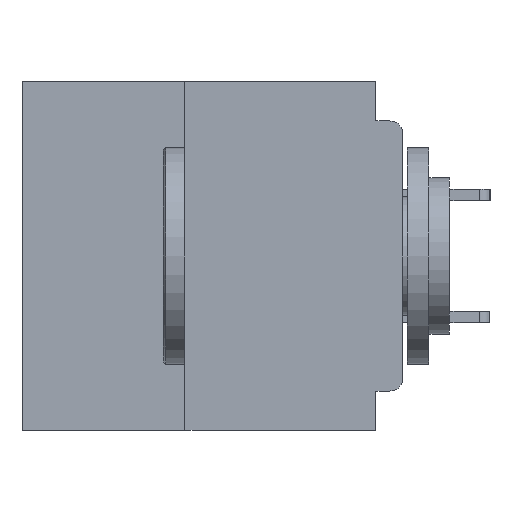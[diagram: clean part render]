
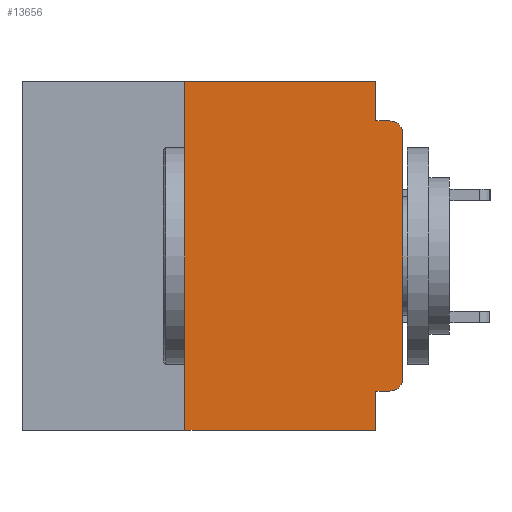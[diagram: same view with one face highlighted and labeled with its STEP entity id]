
A CAD part, left-side view. The second image highlights one B-rep face of the part: STEP entity #13656.
In plain terms, the highlighted planar face has unit normal (-1, 0, 0).
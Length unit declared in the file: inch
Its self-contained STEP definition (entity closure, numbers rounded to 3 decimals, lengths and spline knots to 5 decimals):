
#329 = EDGE_LOOP ( 'NONE', ( #6978, #16661, #8367, #24212, #28486, #1615, #40626, #20095, #39759, #20184 ) ) ;
#485 = LINE ( 'NONE', #35036, #35221 ) ;
#985 = VERTEX_POINT ( 'NONE', #24131 ) ;
#1359 = LINE ( 'NONE', #37734, #35083 ) ;
#1615 = ORIENTED_EDGE ( 'NONE', *, *, #29564, .F. ) ;
#3371 = CIRCLE ( 'NONE', #28947, 0.015 ) ;
#3474 = EDGE_CURVE ( 'NONE', #6209, #32710, #10884, .T. ) ;
#3659 = VERTEX_POINT ( 'NONE', #36518 ) ;
#3709 = DIRECTION ( 'NONE',  ( 0., -1., 0. ) ) ;
#4823 = CARTESIAN_POINT ( 'NONE',  ( 0., 0.437, 0. ) ) ;
#5097 = VECTOR ( 'NONE', #8752, 39.37008 ) ;
#5295 = PLANE ( 'NONE',  #34351 ) ;
#5691 = CARTESIAN_POINT ( 'NONE',  ( 0., 0.031, -0.045 ) ) ;
#5872 = CARTESIAN_POINT ( 'NONE',  ( 0., 0.015, -0.06 ) ) ;
#6209 = VERTEX_POINT ( 'NONE', #13935 ) ;
#6978 = ORIENTED_EDGE ( 'NONE', *, *, #35087, .T. ) ;
#7083 = CARTESIAN_POINT ( 'NONE',  ( 0., 0.015, -0.34 ) ) ;
#7646 = CARTESIAN_POINT ( 'NONE',  ( 0., 0.031, 0. ) ) ;
#8367 = ORIENTED_EDGE ( 'NONE', *, *, #11167, .F. ) ;
#8616 = CARTESIAN_POINT ( 'NONE',  ( 0., 0.031, -0.355 ) ) ;
#8752 = DIRECTION ( 'NONE',  ( 0., -1., 0. ) ) ;
#9049 = VECTOR ( 'NONE', #41411, 39.37008 ) ;
#9162 = DIRECTION ( 'NONE',  ( 0., 0., -1. ) ) ;
#10382 = DIRECTION ( 'NONE',  ( 0., 0., -1. ) ) ;
#10881 = EDGE_CURVE ( 'NONE', #29014, #27771, #3371, .T. ) ;
#10884 = LINE ( 'NONE', #4823, #35881 ) ;
#11167 = EDGE_CURVE ( 'NONE', #37117, #41996, #1359, .T. ) ;
#11799 = CARTESIAN_POINT ( 'NONE',  ( 0., 0.25, -0.4 ) ) ;
#11869 = DIRECTION ( 'NONE',  ( 0., 0., -1. ) ) ;
#13554 = FACE_OUTER_BOUND ( 'NONE', #329, .T. ) ;
#13656 = ADVANCED_FACE ( 'NONE', ( #13554 ), #5295, .F. ) ;
#13844 = LINE ( 'NONE', #40713, #38805 ) ;
#13924 = VECTOR ( 'NONE', #41183, 39.37008 ) ;
#13935 = CARTESIAN_POINT ( 'NONE',  ( 0., 0.25, 0. ) ) ;
#15252 = VECTOR ( 'NONE', #31895, 39.37008 ) ;
#16661 = ORIENTED_EDGE ( 'NONE', *, *, #30199, .T. ) ;
#17846 = EDGE_CURVE ( 'NONE', #21321, #985, #22538, .T. ) ;
#17996 = DIRECTION ( 'NONE',  ( 0., 0., -1. ) ) ;
#18798 = LINE ( 'NONE', #38219, #9049 ) ;
#20095 = ORIENTED_EDGE ( 'NONE', *, *, #23693, .F. ) ;
#20184 = ORIENTED_EDGE ( 'NONE', *, *, #10881, .T. ) ;
#21321 = VERTEX_POINT ( 'NONE', #11799 ) ;
#21367 = AXIS2_PLACEMENT_3D ( 'NONE', #5872, #28768, #9162 ) ;
#21494 = CARTESIAN_POINT ( 'NONE',  ( 0., 0.437, 0. ) ) ;
#21790 = CARTESIAN_POINT ( 'NONE',  ( 0., 0., -0.355 ) ) ;
#22538 = LINE ( 'NONE', #41202, #5097 ) ;
#22633 = VERTEX_POINT ( 'NONE', #8616 ) ;
#23693 = EDGE_CURVE ( 'NONE', #22633, #985, #13844, .T. ) ;
#24131 = CARTESIAN_POINT ( 'NONE',  ( 0., 0.031, -0.4 ) ) ;
#24212 = ORIENTED_EDGE ( 'NONE', *, *, #34505, .F. ) ;
#25039 = LINE ( 'NONE', #35146, #15252 ) ;
#27381 = CIRCLE ( 'NONE', #21367, 0.015 ) ;
#27771 = VERTEX_POINT ( 'NONE', #30484 ) ;
#28104 = DIRECTION ( 'NONE',  ( 0., -1., 0. ) ) ;
#28486 = ORIENTED_EDGE ( 'NONE', *, *, #3474, .F. ) ;
#28550 = DIRECTION ( 'NONE',  ( 0., 0., 1. ) ) ;
#28768 = DIRECTION ( 'NONE',  ( -1., 0., 0. ) ) ;
#28947 = AXIS2_PLACEMENT_3D ( 'NONE', #7083, #29972, #10382 ) ;
#29014 = VERTEX_POINT ( 'NONE', #31547 ) ;
#29564 = EDGE_CURVE ( 'NONE', #21321, #6209, #485, .T. ) ;
#29972 = DIRECTION ( 'NONE',  ( -1., 0., 0. ) ) ;
#30199 = EDGE_CURVE ( 'NONE', #3659, #41996, #27381, .T. ) ;
#30484 = CARTESIAN_POINT ( 'NONE',  ( 0., 0., -0.34 ) ) ;
#31300 = LINE ( 'NONE', #21790, #13924 ) ;
#31547 = CARTESIAN_POINT ( 'NONE',  ( 0., 0.015, -0.355 ) ) ;
#31895 = DIRECTION ( 'NONE',  ( 0., 0., -1. ) ) ;
#32710 = VERTEX_POINT ( 'NONE', #7646 ) ;
#34351 = AXIS2_PLACEMENT_3D ( 'NONE', #21494, #37831, #11869 ) ;
#34505 = EDGE_CURVE ( 'NONE', #32710, #37117, #25039, .T. ) ;
#35036 = CARTESIAN_POINT ( 'NONE',  ( 0., 0.25, -0.4 ) ) ;
#35083 = VECTOR ( 'NONE', #28104, 39.37008 ) ;
#35087 = EDGE_CURVE ( 'NONE', #27771, #3659, #18798, .T. ) ;
#35146 = CARTESIAN_POINT ( 'NONE',  ( 0., 0.031, 0. ) ) ;
#35221 = VECTOR ( 'NONE', #28550, 39.37008 ) ;
#35881 = VECTOR ( 'NONE', #3709, 39.37008 ) ;
#36377 = EDGE_CURVE ( 'NONE', #29014, #22633, #31300, .T. ) ;
#36518 = CARTESIAN_POINT ( 'NONE',  ( 0., 0., -0.06 ) ) ;
#37117 = VERTEX_POINT ( 'NONE', #5691 ) ;
#37734 = CARTESIAN_POINT ( 'NONE',  ( 0., 0., -0.045 ) ) ;
#37831 = DIRECTION ( 'NONE',  ( 1., 0., 0. ) ) ;
#38219 = CARTESIAN_POINT ( 'NONE',  ( 0., 0., 0. ) ) ;
#38805 = VECTOR ( 'NONE', #17996, 39.37008 ) ;
#39007 = CARTESIAN_POINT ( 'NONE',  ( 0., 0.015, -0.045 ) ) ;
#39759 = ORIENTED_EDGE ( 'NONE', *, *, #36377, .F. ) ;
#40626 = ORIENTED_EDGE ( 'NONE', *, *, #17846, .T. ) ;
#40713 = CARTESIAN_POINT ( 'NONE',  ( 0., 0.031, -0.4 ) ) ;
#41183 = DIRECTION ( 'NONE',  ( 0., 1., 0. ) ) ;
#41202 = CARTESIAN_POINT ( 'NONE',  ( 0., 0.437, -0.4 ) ) ;
#41411 = DIRECTION ( 'NONE',  ( 0., 0., 1. ) ) ;
#41996 = VERTEX_POINT ( 'NONE', #39007 ) ;
